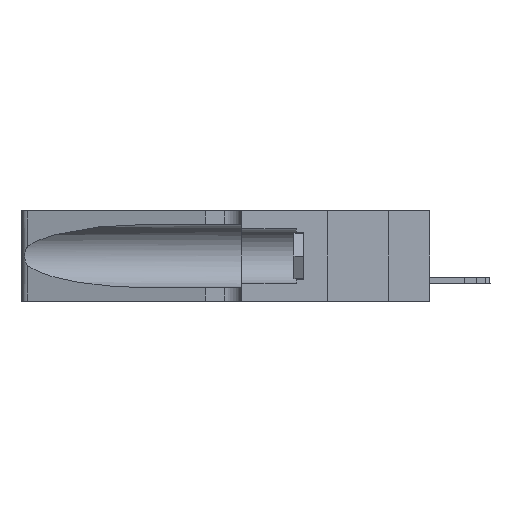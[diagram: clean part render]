
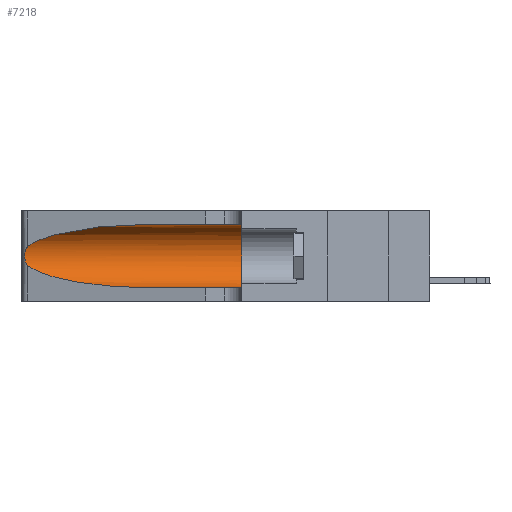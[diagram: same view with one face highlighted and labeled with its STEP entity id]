
A CAD part, left-side view. The second image highlights one B-rep face of the part: STEP entity #7218.
In plain terms, the highlighted cylindrical face has radius 3.308 mm (diameter 6.617 mm), a partial arc.
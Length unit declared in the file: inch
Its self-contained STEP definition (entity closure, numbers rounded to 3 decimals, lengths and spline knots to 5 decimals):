
#810 = ORIENTED_EDGE ( 'NONE', *, *, #15715, .T. ) ;
#1002 = CARTESIAN_POINT ( 'NONE',  ( 0.1305, 0.35, 0.31525 ) ) ;
#1185 = CARTESIAN_POINT ( 'NONE',  ( 0.25854, 1.2359, 0.20912 ) ) ;
#2395 = LINE ( 'NONE', #6507, #14803 ) ;
#3950 = VECTOR ( 'NONE', #14399, 39.37008 ) ;
#4605 = CARTESIAN_POINT ( 'NONE',  ( 0.18966, 0.96281, 0.05475 ) ) ;
#4898 = CARTESIAN_POINT ( 'NONE',  ( 0.26017, 1.23833, 0.17102 ) ) ;
#5063 = EDGE_CURVE ( 'NONE', #14155, #6813, #7690, .T. ) ;
#6507 = CARTESIAN_POINT ( 'NONE',  ( 0.1305, 1.61858, 0.05475 ) ) ;
#6813 = VERTEX_POINT ( 'NONE', #21049 ) ;
#7119 = VERTEX_POINT ( 'NONE', #9226 ) ;
#7218 = ADVANCED_FACE ( 'NONE', ( #14130 ), #19495, .F. ) ;
#7573 = AXIS2_PLACEMENT_3D ( 'NONE', #12787, #14758, #21871 ) ;
#7677 = ORIENTED_EDGE ( 'NONE', *, *, #21439, .F. ) ;
#7690 =( BOUNDED_CURVE ( )  B_SPLINE_CURVE ( 3, ( #18935, #15222, #7835, #18854 ),
 .UNSPECIFIED., .F., .T. ) 
 B_SPLINE_CURVE_WITH_KNOTS ( ( 4, 4 ),
 ( 1.5708, 2.84003 ),
 .UNSPECIFIED. ) 
 CURVE ( )  GEOMETRIC_REPRESENTATION_ITEM ( )  RATIONAL_B_SPLINE_CURVE ( ( 1., 0.87, 0.87, 1. ) ) 
 REPRESENTATION_ITEM ( '' )  );
#7835 = CARTESIAN_POINT ( 'NONE',  ( 0.2373, 1.15595, 0.28018 ) ) ;
#8329 = CARTESIAN_POINT ( 'NONE',  ( 0.1305, 0.72297, 0.31525 ) ) ;
#8686 = CARTESIAN_POINT ( 'NONE',  ( 0.25639, 1.23186, 0.15144 ) ) ;
#9226 = CARTESIAN_POINT ( 'NONE',  ( 0.1305, 0.72297, 0.05475 ) ) ;
#10324 = CARTESIAN_POINT ( 'NONE',  ( 0.26018, 1.23835, 0.19895 ) ) ;
#10344 = EDGE_LOOP ( 'NONE', ( #19340, #16478, #13761, #810, #16888, #7677 ) ) ;
#10449 = CIRCLE ( 'NONE', #7573, 0.13025 ) ;
#10701 = CARTESIAN_POINT ( 'NONE',  ( 0.1305, 1.61858, 0.31525 ) ) ;
#10853 = B_SPLINE_CURVE_WITH_KNOTS ( 'NONE', 3,
 ( #19216, #14089, #12205, #17632, #1185, #10324, #19457, #17552, #4898, #13927, #15579, #8686, #11977, #19295 ),
 .UNSPECIFIED., .F., .F.,
 ( 4, 2, 2, 2, 2, 2, 4 ),
 ( 0., 0.00027, 0.00053, 0.00107, 0.0016, 0.00187, 0.00214 ),
 .UNSPECIFIED. ) ;
#11503 = DIRECTION ( 'NONE',  ( 0., -1., 0. ) ) ;
#11680 = EDGE_CURVE ( 'NONE', #12594, #7119, #20682, .T. ) ;
#11843 = CARTESIAN_POINT ( 'NONE',  ( 0.1305, 0.72297, 0.05475 ) ) ;
#11877 = VERTEX_POINT ( 'NONE', #14779 ) ;
#11977 = CARTESIAN_POINT ( 'NONE',  ( 0.25555, 1.22993, 0.14849 ) ) ;
#12205 = CARTESIAN_POINT ( 'NONE',  ( 0.25639, 1.23184, 0.21858 ) ) ;
#12594 = VERTEX_POINT ( 'NONE', #19082 ) ;
#12787 = CARTESIAN_POINT ( 'NONE',  ( 0.1305, 0.35, 0.185 ) ) ;
#13546 = EDGE_CURVE ( 'NONE', #18078, #11877, #10449, .T. ) ;
#13761 = ORIENTED_EDGE ( 'NONE', *, *, #11680, .T. ) ;
#13793 = CARTESIAN_POINT ( 'NONE',  ( 0.2373, 1.15595, 0.08982 ) ) ;
#13927 = CARTESIAN_POINT ( 'NONE',  ( 0.25856, 1.23593, 0.16098 ) ) ;
#14089 = CARTESIAN_POINT ( 'NONE',  ( 0.25555, 1.22994, 0.2215 ) ) ;
#14130 = FACE_OUTER_BOUND ( 'NONE', #10344, .T. ) ;
#14155 = VERTEX_POINT ( 'NONE', #8329 ) ;
#14399 = DIRECTION ( 'NONE',  ( 0., -1., 0. ) ) ;
#14660 = LINE ( 'NONE', #10701, #3950 ) ;
#14758 = DIRECTION ( 'NONE',  ( 0., 1., 0. ) ) ;
#14779 = CARTESIAN_POINT ( 'NONE',  ( 0.1305, 0.35, 0.05475 ) ) ;
#14786 = DIRECTION ( 'NONE',  ( 0., 0., -1. ) ) ;
#14803 = VECTOR ( 'NONE', #22688, 39.37008 ) ;
#15222 = CARTESIAN_POINT ( 'NONE',  ( 0.18966, 0.96281, 0.31525 ) ) ;
#15299 = CARTESIAN_POINT ( 'NONE',  ( 0.25487, 1.22718, 0.14631 ) ) ;
#15579 = CARTESIAN_POINT ( 'NONE',  ( 0.25789, 1.23486, 0.15765 ) ) ;
#15715 = EDGE_CURVE ( 'NONE', #7119, #11877, #2395, .T. ) ;
#16478 = ORIENTED_EDGE ( 'NONE', *, *, #21232, .T. ) ;
#16888 = ORIENTED_EDGE ( 'NONE', *, *, #13546, .F. ) ;
#17552 = CARTESIAN_POINT ( 'NONE',  ( 0.26075, 1.23896, 0.178 ) ) ;
#17632 = CARTESIAN_POINT ( 'NONE',  ( 0.25787, 1.23484, 0.2124 ) ) ;
#18078 = VERTEX_POINT ( 'NONE', #1002 ) ;
#18854 = CARTESIAN_POINT ( 'NONE',  ( 0.25487, 1.22718, 0.22369 ) ) ;
#18935 = CARTESIAN_POINT ( 'NONE',  ( 0.1305, 0.72297, 0.31525 ) ) ;
#19082 = CARTESIAN_POINT ( 'NONE',  ( 0.25487, 1.22718, 0.14631 ) ) ;
#19216 = CARTESIAN_POINT ( 'NONE',  ( 0.25487, 1.22718, 0.22369 ) ) ;
#19295 = CARTESIAN_POINT ( 'NONE',  ( 0.25487, 1.22718, 0.14631 ) ) ;
#19340 = ORIENTED_EDGE ( 'NONE', *, *, #5063, .T. ) ;
#19457 = CARTESIAN_POINT ( 'NONE',  ( 0.26075, 1.23896, 0.19203 ) ) ;
#19495 = CYLINDRICAL_SURFACE ( 'NONE', #19873, 0.13025 ) ;
#19873 = AXIS2_PLACEMENT_3D ( 'NONE', #22283, #11503, #14786 ) ;
#20682 =( BOUNDED_CURVE ( )  B_SPLINE_CURVE ( 3, ( #15299, #13793, #4605, #11843 ),
 .UNSPECIFIED., .F., .F. ) 
 B_SPLINE_CURVE_WITH_KNOTS ( ( 4, 4 ),
 ( 3.44316, 4.71239 ),
 .UNSPECIFIED. ) 
 CURVE ( )  GEOMETRIC_REPRESENTATION_ITEM ( )  RATIONAL_B_SPLINE_CURVE ( ( 1., 0.87, 0.87, 1. ) ) 
 REPRESENTATION_ITEM ( '' )  );
#21049 = CARTESIAN_POINT ( 'NONE',  ( 0.25487, 1.22718, 0.22369 ) ) ;
#21232 = EDGE_CURVE ( 'NONE', #6813, #12594, #10853, .T. ) ;
#21439 = EDGE_CURVE ( 'NONE', #14155, #18078, #14660, .T. ) ;
#21871 = DIRECTION ( 'NONE',  ( 0., 0., 1. ) ) ;
#22283 = CARTESIAN_POINT ( 'NONE',  ( 0.1305, 1.61858, 0.185 ) ) ;
#22688 = DIRECTION ( 'NONE',  ( 0., -1., 0. ) ) ;
